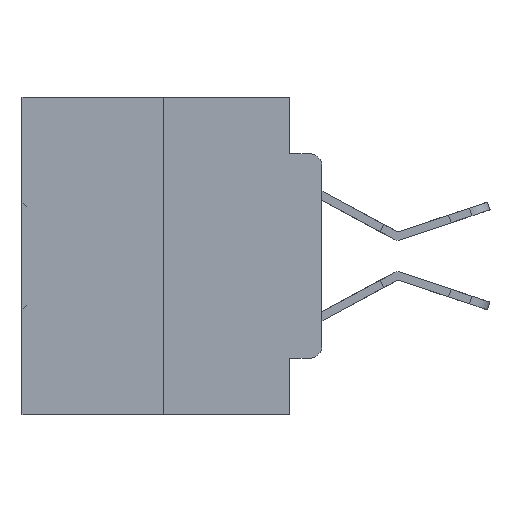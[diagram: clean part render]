
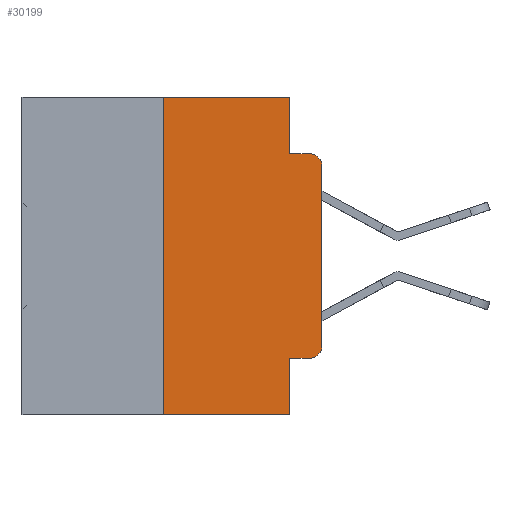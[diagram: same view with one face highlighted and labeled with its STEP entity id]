
A CAD part, left-side view. The second image highlights one B-rep face of the part: STEP entity #30199.
In plain terms, the highlighted planar face has unit normal (-1, 0, 0).
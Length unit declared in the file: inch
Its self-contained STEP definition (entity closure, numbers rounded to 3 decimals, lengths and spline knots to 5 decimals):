
#11 = EDGE_CURVE ( 'NONE', #34382, #30782, #23129, .T. ) ;
#272 = VECTOR ( 'NONE', #2026, 39.37008 ) ;
#366 = LINE ( 'NONE', #5918, #14509 ) ;
#722 = EDGE_CURVE ( 'NONE', #23993, #16373, #366, .T. ) ;
#1777 = DIRECTION ( 'NONE',  ( -1., 0., 0. ) ) ;
#1978 = DIRECTION ( 'NONE',  ( 0., 0., -1. ) ) ;
#2026 = DIRECTION ( 'NONE',  ( 0., 0., -1. ) ) ;
#2677 = CARTESIAN_POINT ( 'NONE',  ( 0., 0.02, -0.4115 ) ) ;
#3009 = CIRCLE ( 'NONE', #29215, 0.02 ) ;
#3334 = EDGE_CURVE ( 'NONE', #20067, #7547, #28826, .T. ) ;
#3346 = VECTOR ( 'NONE', #20782, 39.37008 ) ;
#4053 = CARTESIAN_POINT ( 'NONE',  ( 0., 0., 0. ) ) ;
#4173 = DIRECTION ( 'NONE',  ( 0., 0., -1. ) ) ;
#4506 = EDGE_LOOP ( 'NONE', ( #32254, #18758, #22158, #19190, #33497, #28077, #9631, #33095, #28508, #30616 ) ) ;
#5131 = CARTESIAN_POINT ( 'NONE',  ( 0., 0.25, -0.5 ) ) ;
#5918 = CARTESIAN_POINT ( 'NONE',  ( 0., 0.051, 0. ) ) ;
#5976 = VECTOR ( 'NONE', #21567, 39.37008 ) ;
#6930 = CARTESIAN_POINT ( 'NONE',  ( 0., 0.051, -0.0885 ) ) ;
#7547 = VERTEX_POINT ( 'NONE', #20724 ) ;
#7809 = LINE ( 'NONE', #21539, #272 ) ;
#8315 = EDGE_CURVE ( 'NONE', #11152, #27299, #30103, .T. ) ;
#9022 = EDGE_CURVE ( 'NONE', #16373, #7547, #14349, .T. ) ;
#9256 = VERTEX_POINT ( 'NONE', #25225 ) ;
#9631 = ORIENTED_EDGE ( 'NONE', *, *, #11999, .T. ) ;
#9632 = CARTESIAN_POINT ( 'NONE',  ( 0., 0.473, 0. ) ) ;
#9778 = FACE_OUTER_BOUND ( 'NONE', #4506, .T. ) ;
#9919 = AXIS2_PLACEMENT_3D ( 'NONE', #30096, #30088, #29510 ) ;
#10107 = CARTESIAN_POINT ( 'NONE',  ( 0., 0.25, 0. ) ) ;
#11152 = VERTEX_POINT ( 'NONE', #5131 ) ;
#11600 = CARTESIAN_POINT ( 'NONE',  ( 0., 0.473, -0.5 ) ) ;
#11999 = EDGE_CURVE ( 'NONE', #11152, #9256, #22845, .T. ) ;
#13180 = PLANE ( 'NONE',  #18349 ) ;
#14349 = LINE ( 'NONE', #34928, #5976 ) ;
#14509 = VECTOR ( 'NONE', #4173, 39.37008 ) ;
#15172 = EDGE_CURVE ( 'NONE', #30782, #22877, #3009, .T. ) ;
#16023 = CARTESIAN_POINT ( 'NONE',  ( 0., 0.473, 0. ) ) ;
#16373 = VERTEX_POINT ( 'NONE', #6930 ) ;
#16458 = VECTOR ( 'NONE', #30672, 39.37008 ) ;
#17641 = CARTESIAN_POINT ( 'NONE',  ( 0., 0.051, -0.4115 ) ) ;
#17694 = EDGE_CURVE ( 'NONE', #34382, #9256, #7809, .T. ) ;
#18186 = CARTESIAN_POINT ( 'NONE',  ( 0., 0., -0.3915 ) ) ;
#18258 = LINE ( 'NONE', #4053, #3346 ) ;
#18349 = AXIS2_PLACEMENT_3D ( 'NONE', #16023, #18769, #1978 ) ;
#18527 = DIRECTION ( 'NONE',  ( 0., 0., 1. ) ) ;
#18580 = CARTESIAN_POINT ( 'NONE',  ( 0., 0.02, -0.3915 ) ) ;
#18758 = ORIENTED_EDGE ( 'NONE', *, *, #3334, .T. ) ;
#18769 = DIRECTION ( 'NONE',  ( 1., 0., 0. ) ) ;
#18911 = VECTOR ( 'NONE', #26108, 39.37008 ) ;
#19190 = ORIENTED_EDGE ( 'NONE', *, *, #722, .F. ) ;
#19644 = CARTESIAN_POINT ( 'NONE',  ( 0., 0.25, 0. ) ) ;
#20067 = VERTEX_POINT ( 'NONE', #33128 ) ;
#20291 = EDGE_CURVE ( 'NONE', #27299, #23993, #25274, .T. ) ;
#20724 = CARTESIAN_POINT ( 'NONE',  ( 0., 0.02, -0.0885 ) ) ;
#20782 = DIRECTION ( 'NONE',  ( 0., 0., 1. ) ) ;
#21317 = DIRECTION ( 'NONE',  ( 0., 0., -1. ) ) ;
#21539 = CARTESIAN_POINT ( 'NONE',  ( 0., 0.051, 0. ) ) ;
#21567 = DIRECTION ( 'NONE',  ( 0., -1., 0. ) ) ;
#22158 = ORIENTED_EDGE ( 'NONE', *, *, #9022, .F. ) ;
#22845 = LINE ( 'NONE', #11600, #16458 ) ;
#22877 = VERTEX_POINT ( 'NONE', #18186 ) ;
#23129 = LINE ( 'NONE', #17641, #29407 ) ;
#23993 = VERTEX_POINT ( 'NONE', #26059 ) ;
#25225 = CARTESIAN_POINT ( 'NONE',  ( 0., 0.051, -0.5 ) ) ;
#25274 = LINE ( 'NONE', #9632, #18911 ) ;
#26059 = CARTESIAN_POINT ( 'NONE',  ( 0., 0.051, 0. ) ) ;
#26108 = DIRECTION ( 'NONE',  ( 0., -1., 0. ) ) ;
#27299 = VERTEX_POINT ( 'NONE', #19644 ) ;
#28077 = ORIENTED_EDGE ( 'NONE', *, *, #8315, .F. ) ;
#28508 = ORIENTED_EDGE ( 'NONE', *, *, #11, .T. ) ;
#28826 = CIRCLE ( 'NONE', #9919, 0.02 ) ;
#29215 = AXIS2_PLACEMENT_3D ( 'NONE', #18580, #1777, #21317 ) ;
#29407 = VECTOR ( 'NONE', #30537, 39.37008 ) ;
#29510 = DIRECTION ( 'NONE',  ( 0., 0., -1. ) ) ;
#30088 = DIRECTION ( 'NONE',  ( -1., 0., 0. ) ) ;
#30096 = CARTESIAN_POINT ( 'NONE',  ( 0., 0.02, -0.1085 ) ) ;
#30103 = LINE ( 'NONE', #10107, #35508 ) ;
#30199 = ADVANCED_FACE ( 'NONE', ( #9778 ), #13180, .F. ) ;
#30537 = DIRECTION ( 'NONE',  ( 0., -1., 0. ) ) ;
#30616 = ORIENTED_EDGE ( 'NONE', *, *, #15172, .T. ) ;
#30672 = DIRECTION ( 'NONE',  ( 0., -1., 0. ) ) ;
#30782 = VERTEX_POINT ( 'NONE', #2677 ) ;
#32254 = ORIENTED_EDGE ( 'NONE', *, *, #34143, .T. ) ;
#32401 = CARTESIAN_POINT ( 'NONE',  ( 0., 0.051, -0.4115 ) ) ;
#33095 = ORIENTED_EDGE ( 'NONE', *, *, #17694, .F. ) ;
#33128 = CARTESIAN_POINT ( 'NONE',  ( 0., 0., -0.1085 ) ) ;
#33497 = ORIENTED_EDGE ( 'NONE', *, *, #20291, .F. ) ;
#34143 = EDGE_CURVE ( 'NONE', #22877, #20067, #18258, .T. ) ;
#34382 = VERTEX_POINT ( 'NONE', #32401 ) ;
#34928 = CARTESIAN_POINT ( 'NONE',  ( 0., 0.051, -0.0885 ) ) ;
#35508 = VECTOR ( 'NONE', #18527, 39.37008 ) ;
